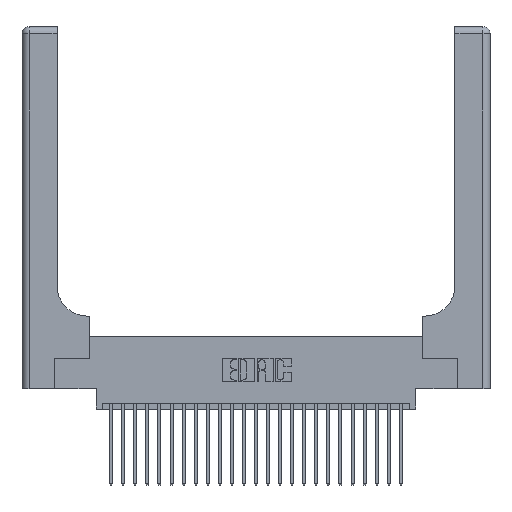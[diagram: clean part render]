
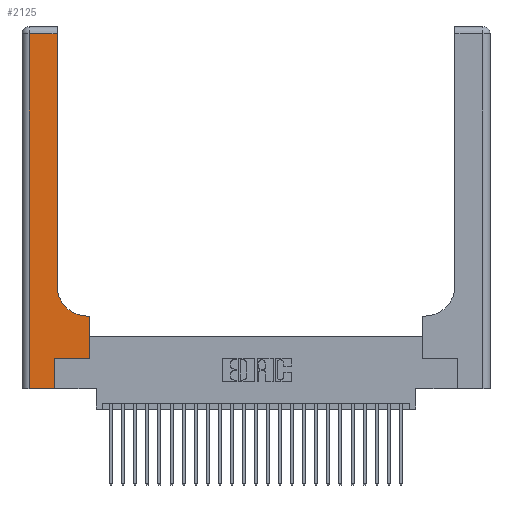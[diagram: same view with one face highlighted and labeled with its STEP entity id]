
A CAD part, top view. The second image highlights one B-rep face of the part: STEP entity #2125.
In plain terms, the highlighted planar face has unit normal (0, 0, 1).
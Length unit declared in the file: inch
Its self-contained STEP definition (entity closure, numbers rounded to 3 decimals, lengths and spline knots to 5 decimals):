
#203 = ORIENTED_EDGE ( 'NONE', *, *, #24527, .T. ) ;
#851 = VERTEX_POINT ( 'NONE', #11417 ) ;
#875 = CARTESIAN_POINT ( 'NONE',  ( 0.06, 0., 0.37 ) ) ;
#1013 = CARTESIAN_POINT ( 'NONE',  ( 0., 0., 0.37 ) ) ;
#1082 = PLANE ( 'NONE',  #7248 ) ;
#1408 = EDGE_LOOP ( 'NONE', ( #13898, #13316, #12410, #12459, #7653, #25927, #18530, #203, #13905 ) ) ;
#1451 = DIRECTION ( 'NONE',  ( 0., 0., -1. ) ) ;
#1590 = VERTEX_POINT ( 'NONE', #18614 ) ;
#2125 = ADVANCED_FACE ( 'NONE', ( #17418 ), #1082, .F. ) ;
#2711 = VERTEX_POINT ( 'NONE', #4997 ) ;
#2755 = CARTESIAN_POINT ( 'NONE',  ( 0.5415, 0.85, 0.37 ) ) ;
#3237 = DIRECTION ( 'NONE',  ( -1., 0., 0. ) ) ;
#3668 = EDGE_CURVE ( 'NONE', #851, #10638, #27167, .T. ) ;
#4038 = EDGE_CURVE ( 'NONE', #2711, #21443, #16568, .T. ) ;
#4443 = CARTESIAN_POINT ( 'NONE',  ( 0.5585, 0.25, 0.37 ) ) ;
#4584 = EDGE_CURVE ( 'NONE', #10638, #17936, #25131, .T. ) ;
#4714 = DIRECTION ( 'NONE',  ( 0., 1., 0. ) ) ;
#4997 = CARTESIAN_POINT ( 'NONE',  ( 0.06, 2.94, 0.37 ) ) ;
#5115 = LINE ( 'NONE', #8576, #14294 ) ;
#5319 = DIRECTION ( 'NONE',  ( -1., 0., 0. ) ) ;
#5968 = VECTOR ( 'NONE', #13642, 39.37008 ) ;
#7248 = AXIS2_PLACEMENT_3D ( 'NONE', #24599, #1451, #5319 ) ;
#7653 = ORIENTED_EDGE ( 'NONE', *, *, #24168, .T. ) ;
#8576 = CARTESIAN_POINT ( 'NONE',  ( 0.269, 0., 0.37 ) ) ;
#10295 = CARTESIAN_POINT ( 'NONE',  ( 0.269, 0., 0.37 ) ) ;
#10529 = DIRECTION ( 'NONE',  ( 1., 0., 0. ) ) ;
#10626 = CARTESIAN_POINT ( 'NONE',  ( 0.269, 0.25, 0.37 ) ) ;
#10638 = VERTEX_POINT ( 'NONE', #26582 ) ;
#11402 = DIRECTION ( 'NONE',  ( 1., 0., 0. ) ) ;
#11417 = CARTESIAN_POINT ( 'NONE',  ( 0.5415, 0.6, 0.37 ) ) ;
#11559 = LINE ( 'NONE', #20242, #5968 ) ;
#12044 = CARTESIAN_POINT ( 'NONE',  ( 0.5585, 0.6, 0.37 ) ) ;
#12319 = VECTOR ( 'NONE', #10529, 39.37008 ) ;
#12410 = ORIENTED_EDGE ( 'NONE', *, *, #4038, .T. ) ;
#12459 = ORIENTED_EDGE ( 'NONE', *, *, #16636, .T. ) ;
#13316 = ORIENTED_EDGE ( 'NONE', *, *, #16065, .T. ) ;
#13430 = EDGE_CURVE ( 'NONE', #17829, #18081, #24217, .T. ) ;
#13607 = CARTESIAN_POINT ( 'NONE',  ( 0.2915, 0.6, 0.37 ) ) ;
#13642 = DIRECTION ( 'NONE',  ( -1., 0., 0. ) ) ;
#13829 = LINE ( 'NONE', #1013, #18097 ) ;
#13898 = ORIENTED_EDGE ( 'NONE', *, *, #4584, .T. ) ;
#13905 = ORIENTED_EDGE ( 'NONE', *, *, #3668, .T. ) ;
#14197 = CARTESIAN_POINT ( 'NONE',  ( 0.06, 3., 0.37 ) ) ;
#14294 = VECTOR ( 'NONE', #25379, 39.37008 ) ;
#16065 = EDGE_CURVE ( 'NONE', #17936, #2711, #11559, .T. ) ;
#16568 = LINE ( 'NONE', #14197, #20847 ) ;
#16636 = EDGE_CURVE ( 'NONE', #21443, #18213, #13829, .T. ) ;
#17248 = LINE ( 'NONE', #13607, #23164 ) ;
#17418 = FACE_OUTER_BOUND ( 'NONE', #1408, .T. ) ;
#17529 = DIRECTION ( 'NONE',  ( 0., 0., -1. ) ) ;
#17829 = VERTEX_POINT ( 'NONE', #21552 ) ;
#17936 = VERTEX_POINT ( 'NONE', #18354 ) ;
#18081 = VERTEX_POINT ( 'NONE', #12044 ) ;
#18097 = VECTOR ( 'NONE', #11402, 39.37008 ) ;
#18213 = VERTEX_POINT ( 'NONE', #10295 ) ;
#18354 = CARTESIAN_POINT ( 'NONE',  ( 0.2915, 2.94, 0.37 ) ) ;
#18530 = ORIENTED_EDGE ( 'NONE', *, *, #13430, .T. ) ;
#18549 = VECTOR ( 'NONE', #18571, 39.37008 ) ;
#18571 = DIRECTION ( 'NONE',  ( 0., 1., 0. ) ) ;
#18614 = CARTESIAN_POINT ( 'NONE',  ( 0.269, 0.25, 0.37 ) ) ;
#20242 = CARTESIAN_POINT ( 'NONE',  ( 0., 2.94, 0.37 ) ) ;
#20629 = EDGE_CURVE ( 'NONE', #1590, #17829, #22843, .T. ) ;
#20847 = VECTOR ( 'NONE', #24596, 39.37008 ) ;
#21443 = VERTEX_POINT ( 'NONE', #875 ) ;
#21552 = CARTESIAN_POINT ( 'NONE',  ( 0.5585, 0.25, 0.37 ) ) ;
#22843 = LINE ( 'NONE', #10626, #12319 ) ;
#23164 = VECTOR ( 'NONE', #3237, 39.37008 ) ;
#23798 = DIRECTION ( 'NONE',  ( 1., 0., 0. ) ) ;
#24168 = EDGE_CURVE ( 'NONE', #18213, #1590, #5115, .T. ) ;
#24217 = LINE ( 'NONE', #4443, #24876 ) ;
#24527 = EDGE_CURVE ( 'NONE', #18081, #851, #17248, .T. ) ;
#24596 = DIRECTION ( 'NONE',  ( 0., -1., 0. ) ) ;
#24599 = CARTESIAN_POINT ( 'NONE',  ( 0., 3., 0.37 ) ) ;
#24876 = VECTOR ( 'NONE', #4714, 39.37008 ) ;
#24996 = AXIS2_PLACEMENT_3D ( 'NONE', #2755, #17529, #23798 ) ;
#25131 = LINE ( 'NONE', #26245, #18549 ) ;
#25379 = DIRECTION ( 'NONE',  ( 0., 1., 0. ) ) ;
#25927 = ORIENTED_EDGE ( 'NONE', *, *, #20629, .T. ) ;
#26245 = CARTESIAN_POINT ( 'NONE',  ( 0.2915, 3., 0.37 ) ) ;
#26582 = CARTESIAN_POINT ( 'NONE',  ( 0.2915, 0.85, 0.37 ) ) ;
#27167 = CIRCLE ( 'NONE', #24996, 0.25 ) ;
